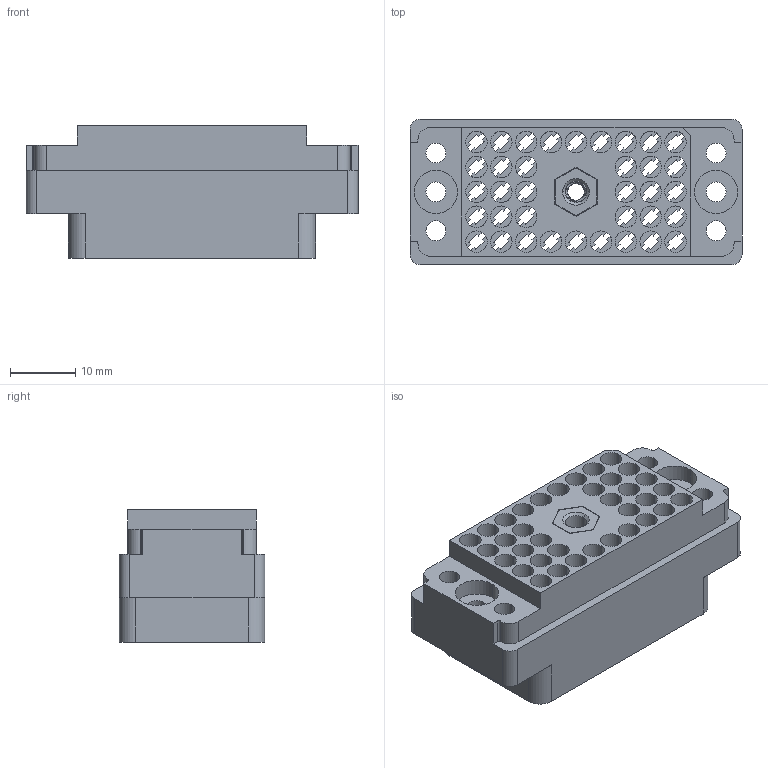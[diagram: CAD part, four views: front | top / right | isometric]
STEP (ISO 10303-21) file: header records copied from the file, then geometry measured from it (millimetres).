
FILE_DESCRIPTION (( 'STEP AP203' ), '1' );
FILE_NAME ('519-036-000-306.STEP', '2020-03-02T21:17:18', ( '' ), ( '' ), 'SwSTEP 2.0', 'SolidWorks 2016', '' );
FILE_SCHEMA (( 'CONFIG_CONTROL_DESIGN' ));
Length unit declared in the file: inch
Products named in the file (3): 519 Plug Insulator_036; 519-036-000-306; 516-252-035-100_516-252-035-100
Assembly tree (2 placements, depth 2):
  519-036-000-306
    519 Plug Insulator_036
    516-252-035-100_516-252-035-100
Bounding box: 50.8 x 22.25 x 20.27 mm (x, y, z)
Volume: 9051.6 mm3; surface area: 11756.6 mm2
Topology: 2 solids, 2 shells, 908 faces, 2645 edges, 1760 vertices
Faces by surface type: plane 626, cylinder 264, cone 12, bspline 6
Entity records: 32788 total; most frequent: CARTESIAN_POINT 7764, ORIENTED_EDGE 5290, DIRECTION 5069, EDGE_CURVE 2645, VECTOR 1935, LINE 1935, VERTEX_POINT 1760, AXIS2_PLACEMENT_3D 1567
